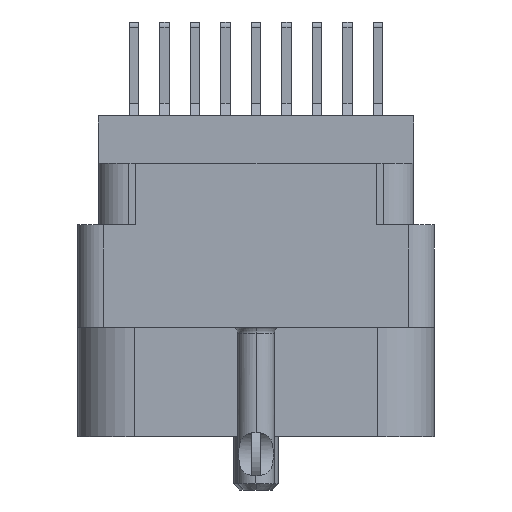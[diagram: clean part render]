
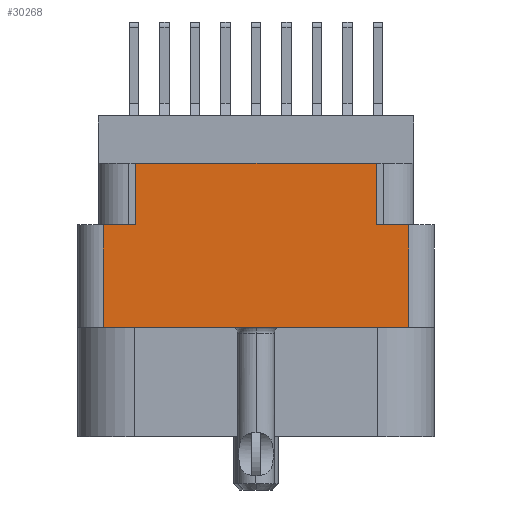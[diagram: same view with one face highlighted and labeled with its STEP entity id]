
A CAD part, left-side view. The second image highlights one B-rep face of the part: STEP entity #30268.
In plain terms, the highlighted planar face has unit normal (-1, 0, 0).
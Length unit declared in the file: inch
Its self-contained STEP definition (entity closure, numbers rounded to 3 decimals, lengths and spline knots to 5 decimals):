
#1761 = EDGE_CURVE ( 'NONE', #40417, #19922, #27953, .T. ) ;
#3166 = DIRECTION ( 'NONE',  ( 0., 0., 1. ) ) ;
#3324 = DIRECTION ( 'NONE',  ( -1., 0., 0. ) ) ;
#5785 = VECTOR ( 'NONE', #40479, 39.37008 ) ;
#6225 = VERTEX_POINT ( 'NONE', #19941 ) ;
#6374 = ORIENTED_EDGE ( 'NONE', *, *, #6660, .F. ) ;
#6660 = EDGE_CURVE ( 'NONE', #19922, #9003, #11677, .T. ) ;
#8873 = ORIENTED_EDGE ( 'NONE', *, *, #46215, .T. ) ;
#9003 = VERTEX_POINT ( 'NONE', #20591 ) ;
#9678 = LINE ( 'NONE', #29459, #23387 ) ;
#10614 = ORIENTED_EDGE ( 'NONE', *, *, #23445, .F. ) ;
#10651 = DIRECTION ( 'NONE',  ( 0., -1., 0. ) ) ;
#10908 = ORIENTED_EDGE ( 'NONE', *, *, #40085, .T. ) ;
#11514 = DIRECTION ( 'NONE',  ( 0., -1., 0. ) ) ;
#11677 = LINE ( 'NONE', #37868, #25334 ) ;
#13196 = ORIENTED_EDGE ( 'NONE', *, *, #1761, .F. ) ;
#14661 = CARTESIAN_POINT ( 'NONE',  ( -1., -0.438, -0.789 ) ) ;
#15772 = CARTESIAN_POINT ( 'NONE',  ( -1., 0.296, -0.268 ) ) ;
#15924 = DIRECTION ( 'NONE',  ( 0., 0., 1. ) ) ;
#16874 = VERTEX_POINT ( 'NONE', #19076 ) ;
#16989 = AXIS2_PLACEMENT_3D ( 'NONE', #14661, #3324, #3166 ) ;
#17040 = CARTESIAN_POINT ( 'NONE',  ( -1., 0.296, -0.117 ) ) ;
#17162 = FACE_OUTER_BOUND ( 'NONE', #40991, .T. ) ;
#18125 = VECTOR ( 'NONE', #33559, 39.37008 ) ;
#18472 = DIRECTION ( 'NONE',  ( 0., 0., 1. ) ) ;
#18782 = ORIENTED_EDGE ( 'NONE', *, *, #37839, .T. ) ;
#18786 = DIRECTION ( 'NONE',  ( 0., -1., 0. ) ) ;
#19060 = CARTESIAN_POINT ( 'NONE',  ( -1., -0.376, -0.52 ) ) ;
#19076 = CARTESIAN_POINT ( 'NONE',  ( -1., 0.376, -0.268 ) ) ;
#19922 = VERTEX_POINT ( 'NONE', #17040 ) ;
#19941 = CARTESIAN_POINT ( 'NONE',  ( -1., -0.376, -0.268 ) ) ;
#20487 = CARTESIAN_POINT ( 'NONE',  ( -1., -0.296, -0.268 ) ) ;
#20591 = CARTESIAN_POINT ( 'NONE',  ( -1., -0.296, -0.117 ) ) ;
#21151 = LINE ( 'NONE', #44775, #5785 ) ;
#23387 = VECTOR ( 'NONE', #11514, 39.37008 ) ;
#23445 = EDGE_CURVE ( 'NONE', #16874, #40417, #30134, .T. ) ;
#25334 = VECTOR ( 'NONE', #18786, 39.37008 ) ;
#25881 = VERTEX_POINT ( 'NONE', #20487 ) ;
#26001 = EDGE_CURVE ( 'NONE', #26331, #6225, #27197, .T. ) ;
#26331 = VERTEX_POINT ( 'NONE', #19060 ) ;
#27197 = LINE ( 'NONE', #37422, #18125 ) ;
#27364 = CARTESIAN_POINT ( 'NONE',  ( -1., 0.296, -0.268 ) ) ;
#27953 = LINE ( 'NONE', #15772, #41430 ) ;
#28989 = VECTOR ( 'NONE', #10651, 39.37008 ) ;
#29459 = CARTESIAN_POINT ( 'NONE',  ( -1., 0., -0.268 ) ) ;
#30134 = LINE ( 'NONE', #39910, #28989 ) ;
#30268 = ADVANCED_FACE ( 'NONE', ( #17162 ), #44200, .T. ) ;
#30785 = VECTOR ( 'NONE', #18472, 39.37008 ) ;
#31046 = ORIENTED_EDGE ( 'NONE', *, *, #26001, .T. ) ;
#31103 = EDGE_CURVE ( 'NONE', #25881, #6225, #9678, .T. ) ;
#32310 = CARTESIAN_POINT ( 'NONE',  ( -1., 0., -0.52 ) ) ;
#32468 = DIRECTION ( 'NONE',  ( 0., -1., 0. ) ) ;
#33103 = LINE ( 'NONE', #40077, #30785 ) ;
#33559 = DIRECTION ( 'NONE',  ( 0., 0., 1. ) ) ;
#34665 = ORIENTED_EDGE ( 'NONE', *, *, #31103, .F. ) ;
#35446 = VERTEX_POINT ( 'NONE', #44391 ) ;
#37422 = CARTESIAN_POINT ( 'NONE',  ( -1., -0.376, -0.789 ) ) ;
#37839 = EDGE_CURVE ( 'NONE', #16874, #35446, #21151, .T. ) ;
#37868 = CARTESIAN_POINT ( 'NONE',  ( -1., 0.438, -0.117 ) ) ;
#39910 = CARTESIAN_POINT ( 'NONE',  ( -1., 0., -0.268 ) ) ;
#40077 = CARTESIAN_POINT ( 'NONE',  ( -1., -0.296, -0.268 ) ) ;
#40085 = EDGE_CURVE ( 'NONE', #35446, #26331, #45829, .T. ) ;
#40417 = VERTEX_POINT ( 'NONE', #27364 ) ;
#40479 = DIRECTION ( 'NONE',  ( 0., 0., -1. ) ) ;
#40991 = EDGE_LOOP ( 'NONE', ( #10614, #18782, #10908, #31046, #34665, #8873, #6374, #13196 ) ) ;
#41430 = VECTOR ( 'NONE', #15924, 39.37008 ) ;
#41890 = VECTOR ( 'NONE', #32468, 39.37008 ) ;
#44200 = PLANE ( 'NONE',  #16989 ) ;
#44391 = CARTESIAN_POINT ( 'NONE',  ( -1., 0.376, -0.52 ) ) ;
#44775 = CARTESIAN_POINT ( 'NONE',  ( -1., 0.376, -0.789 ) ) ;
#45829 = LINE ( 'NONE', #32310, #41890 ) ;
#46215 = EDGE_CURVE ( 'NONE', #25881, #9003, #33103, .T. ) ;
